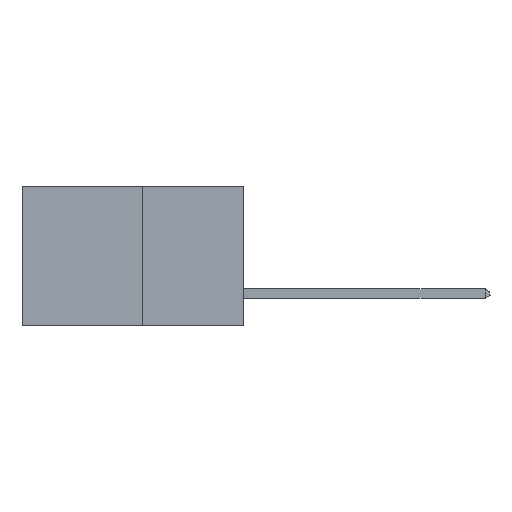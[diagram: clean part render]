
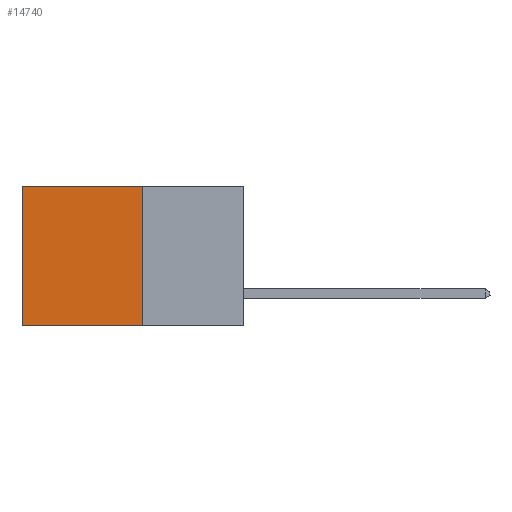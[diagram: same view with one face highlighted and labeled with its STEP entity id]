
A CAD part, left-side view. The second image highlights one B-rep face of the part: STEP entity #14740.
In plain terms, the highlighted planar face has unit normal (-1, 0, 0).
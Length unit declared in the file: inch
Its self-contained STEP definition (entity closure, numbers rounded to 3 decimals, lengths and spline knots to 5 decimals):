
#502 = FACE_OUTER_BOUND ( 'NONE', #11867, .T. ) ;
#884 = EDGE_CURVE ( 'NONE', #15836, #1306, #9103, .T. ) ;
#1306 = VERTEX_POINT ( 'NONE', #1347 ) ;
#1347 = CARTESIAN_POINT ( 'NONE',  ( 0.277, 0.59, 0. ) ) ;
#1674 = VECTOR ( 'NONE', #10341, 39.37008 ) ;
#1715 = VERTEX_POINT ( 'NONE', #5233 ) ;
#2900 = DIRECTION ( 'NONE',  ( 0., 0., -1. ) ) ;
#2937 = CARTESIAN_POINT ( 'NONE',  ( 0.277, 0.27, -0.37 ) ) ;
#3020 = VECTOR ( 'NONE', #2900, 39.37008 ) ;
#3242 = CARTESIAN_POINT ( 'NONE',  ( 0.277, 0.27, -0.37 ) ) ;
#4139 = ORIENTED_EDGE ( 'NONE', *, *, #4229, .T. ) ;
#4229 = EDGE_CURVE ( 'NONE', #1306, #1715, #13263, .T. ) ;
#4711 = EDGE_CURVE ( 'NONE', #15836, #11460, #9609, .T. ) ;
#4813 = VECTOR ( 'NONE', #9231, 39.37008 ) ;
#5233 = CARTESIAN_POINT ( 'NONE',  ( 0.277, 0.59, -0.37 ) ) ;
#5658 = ORIENTED_EDGE ( 'NONE', *, *, #4711, .F. ) ;
#5675 = CARTESIAN_POINT ( 'NONE',  ( 0.277, 0.27, -0.37 ) ) ;
#5965 = CARTESIAN_POINT ( 'NONE',  ( 0.277, 0.27, 0. ) ) ;
#6895 = DIRECTION ( 'NONE',  ( 0., 1., 0. ) ) ;
#6915 = DIRECTION ( 'NONE',  ( 0., 0., -1. ) ) ;
#8106 = LINE ( 'NONE', #11713, #4813 ) ;
#8600 = ORIENTED_EDGE ( 'NONE', *, *, #15444, .F. ) ;
#9103 = LINE ( 'NONE', #5965, #11985 ) ;
#9231 = DIRECTION ( 'NONE',  ( 0., 1., 0. ) ) ;
#9609 = LINE ( 'NONE', #2937, #3020 ) ;
#9673 = AXIS2_PLACEMENT_3D ( 'NONE', #5675, #14234, #6915 ) ;
#10341 = DIRECTION ( 'NONE',  ( 0., 0., -1. ) ) ;
#10349 = CARTESIAN_POINT ( 'NONE',  ( 0.277, 0.59, -0.37 ) ) ;
#11460 = VERTEX_POINT ( 'NONE', #3242 ) ;
#11713 = CARTESIAN_POINT ( 'NONE',  ( 0.277, 0.27, -0.37 ) ) ;
#11867 = EDGE_LOOP ( 'NONE', ( #4139, #8600, #5658, #13590 ) ) ;
#11985 = VECTOR ( 'NONE', #6895, 39.37008 ) ;
#12996 = PLANE ( 'NONE',  #9673 ) ;
#13263 = LINE ( 'NONE', #10349, #1674 ) ;
#13590 = ORIENTED_EDGE ( 'NONE', *, *, #884, .T. ) ;
#13606 = CARTESIAN_POINT ( 'NONE',  ( 0.277, 0.27, 0. ) ) ;
#14234 = DIRECTION ( 'NONE',  ( 1., 0., 0. ) ) ;
#14740 = ADVANCED_FACE ( 'NONE', ( #502 ), #12996, .F. ) ;
#15444 = EDGE_CURVE ( 'NONE', #11460, #1715, #8106, .T. ) ;
#15836 = VERTEX_POINT ( 'NONE', #13606 ) ;
